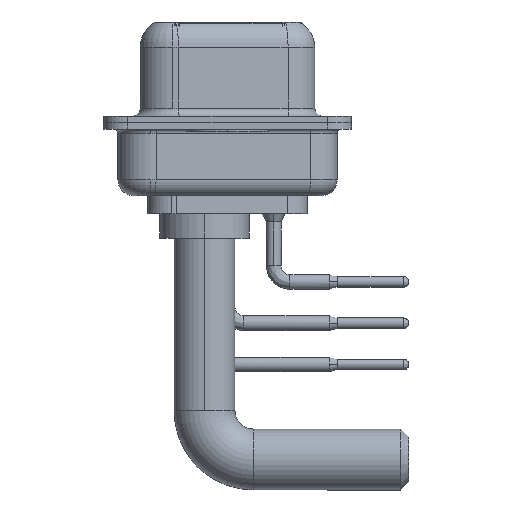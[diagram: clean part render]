
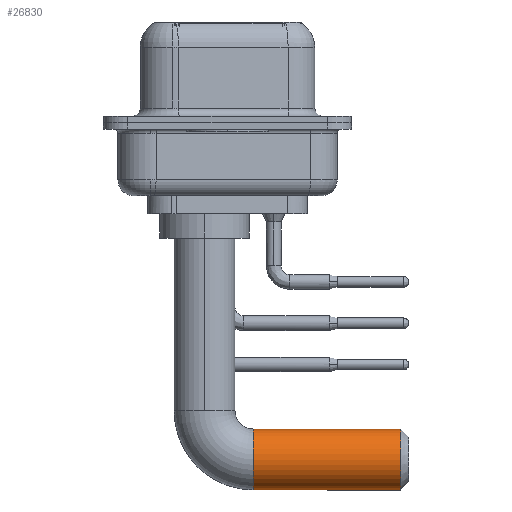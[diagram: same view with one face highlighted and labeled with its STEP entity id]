
A CAD part, left-side view. The second image highlights one B-rep face of the part: STEP entity #26830.
In plain terms, the highlighted cylindrical face has radius 1.875 mm (diameter 3.75 mm), a partial arc.
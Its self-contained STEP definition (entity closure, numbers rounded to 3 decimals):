
#94 = DIRECTION ( 'NONE',  ( 0., -1., 0. ) ) ;
#479 = ORIENTED_EDGE ( 'NONE', *, *, #26623, .T. ) ;
#2130 = DIRECTION ( 'NONE',  ( 0., -1., 0. ) ) ;
#5767 = AXIS2_PLACEMENT_3D ( 'NONE', #24510, #18067, #15968 ) ;
#6364 = ORIENTED_EDGE ( 'NONE', *, *, #26381, .T. ) ;
#7666 = VERTEX_POINT ( 'NONE', #13282 ) ;
#8067 = AXIS2_PLACEMENT_3D ( 'NONE', #10391, #94, #8297 ) ;
#8297 = DIRECTION ( 'NONE',  ( 0., 0., -1. ) ) ;
#8472 = DIRECTION ( 'NONE',  ( 0., -1., 0. ) ) ;
#8873 = ORIENTED_EDGE ( 'NONE', *, *, #15916, .T. ) ;
#9389 = AXIS2_PLACEMENT_3D ( 'NONE', #12650, #8472, #25222 ) ;
#10384 = CARTESIAN_POINT ( 'NONE',  ( 0., -12.07, -11.755 ) ) ;
#10391 = CARTESIAN_POINT ( 'NONE',  ( 0., -3., -13.63 ) ) ;
#10966 = CARTESIAN_POINT ( 'NONE',  ( 0., -3., -15.505 ) ) ;
#11104 = LINE ( 'NONE', #10966, #12959 ) ;
#12338 = FACE_OUTER_BOUND ( 'NONE', #16566, .T. ) ;
#12650 = CARTESIAN_POINT ( 'NONE',  ( 0., -3., -13.63 ) ) ;
#12959 = VECTOR ( 'NONE', #19467, 1000. ) ;
#13282 = CARTESIAN_POINT ( 'NONE',  ( 0., -12.07, -15.505 ) ) ;
#15916 = EDGE_CURVE ( 'NONE', #7666, #24271, #25364, .T. ) ;
#15968 = DIRECTION ( 'NONE',  ( 0., 0., -1. ) ) ;
#16444 = CARTESIAN_POINT ( 'NONE',  ( 0., -3., -11.755 ) ) ;
#16566 = EDGE_LOOP ( 'NONE', ( #26249, #6364, #479, #8873 ) ) ;
#16796 = EDGE_CURVE ( 'NONE', #24801, #24271, #16858, .T. ) ;
#16858 = LINE ( 'NONE', #16444, #24523 ) ;
#18067 = DIRECTION ( 'NONE',  ( 0., 1., 0. ) ) ;
#19165 = CYLINDRICAL_SURFACE ( 'NONE', #8067, 1.875 ) ;
#19467 = DIRECTION ( 'NONE',  ( 0., -1., 0. ) ) ;
#20930 = CIRCLE ( 'NONE', #9389, 1.875 ) ;
#21849 = CARTESIAN_POINT ( 'NONE',  ( 0., -3., -15.505 ) ) ;
#24271 = VERTEX_POINT ( 'NONE', #10384 ) ;
#24510 = CARTESIAN_POINT ( 'NONE',  ( 0., -12.07, -13.63 ) ) ;
#24523 = VECTOR ( 'NONE', #2130, 1000. ) ;
#24801 = VERTEX_POINT ( 'NONE', #26206 ) ;
#25222 = DIRECTION ( 'NONE',  ( -1., 0., 0. ) ) ;
#25364 = CIRCLE ( 'NONE', #5767, 1.875 ) ;
#26206 = CARTESIAN_POINT ( 'NONE',  ( 0., -3., -11.755 ) ) ;
#26249 = ORIENTED_EDGE ( 'NONE', *, *, #16796, .F. ) ;
#26381 = EDGE_CURVE ( 'NONE', #24801, #26500, #20930, .T. ) ;
#26500 = VERTEX_POINT ( 'NONE', #21849 ) ;
#26623 = EDGE_CURVE ( 'NONE', #26500, #7666, #11104, .T. ) ;
#26830 = ADVANCED_FACE ( 'NONE', ( #12338 ), #19165, .T. ) ;
